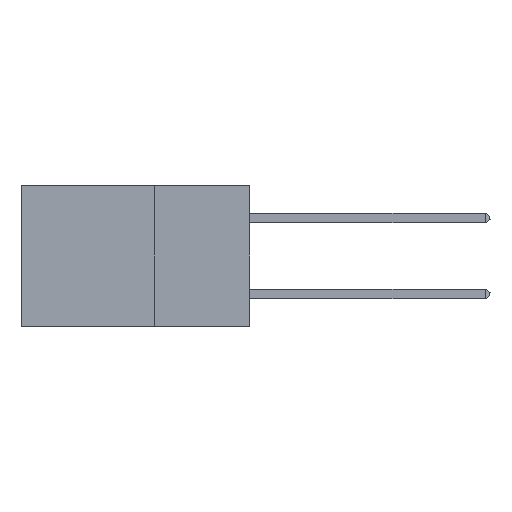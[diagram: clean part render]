
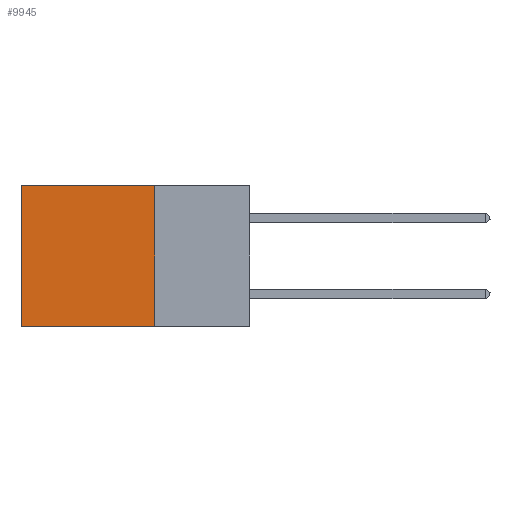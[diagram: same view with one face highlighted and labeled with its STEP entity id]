
A CAD part, left-side view. The second image highlights one B-rep face of the part: STEP entity #9945.
In plain terms, the highlighted planar face has unit normal (-1, 0, 0).
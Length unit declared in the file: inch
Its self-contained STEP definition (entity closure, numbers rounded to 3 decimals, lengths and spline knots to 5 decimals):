
#207 = EDGE_CURVE ( 'NONE', #21221, #17875, #10929, .T. ) ;
#792 = DIRECTION ( 'NONE',  ( 0., 0., -1. ) ) ;
#2050 = AXIS2_PLACEMENT_3D ( 'NONE', #10026, #14637, #792 ) ;
#2463 = ORIENTED_EDGE ( 'NONE', *, *, #19929, .F. ) ;
#3880 = ORIENTED_EDGE ( 'NONE', *, *, #20287, .T. ) ;
#4412 = EDGE_CURVE ( 'NONE', #27515, #17875, #10033, .T. ) ;
#4628 = CARTESIAN_POINT ( 'NONE',  ( 0.2875, 0.6, 0. ) ) ;
#6658 = CARTESIAN_POINT ( 'NONE',  ( 0.2875, 0.25, 0. ) ) ;
#7528 = ORIENTED_EDGE ( 'NONE', *, *, #207, .T. ) ;
#7703 = PLANE ( 'NONE',  #2050 ) ;
#9314 = VECTOR ( 'NONE', #17107, 39.37008 ) ;
#9533 = FACE_OUTER_BOUND ( 'NONE', #23847, .T. ) ;
#9945 = ADVANCED_FACE ( 'NONE', ( #9533 ), #7703, .F. ) ;
#10026 = CARTESIAN_POINT ( 'NONE',  ( 0.2875, 0.25, 0. ) ) ;
#10033 = LINE ( 'NONE', #15262, #15445 ) ;
#10579 = CARTESIAN_POINT ( 'NONE',  ( 0.2875, 0.25, -0.37 ) ) ;
#10929 = LINE ( 'NONE', #4628, #22416 ) ;
#11270 = DIRECTION ( 'NONE',  ( 0., 0., -1. ) ) ;
#12672 = VERTEX_POINT ( 'NONE', #23193 ) ;
#13256 = VECTOR ( 'NONE', #11270, 39.37008 ) ;
#14637 = DIRECTION ( 'NONE',  ( 1., 0., 0. ) ) ;
#15262 = CARTESIAN_POINT ( 'NONE',  ( 0.2875, 0.25, -0.37 ) ) ;
#15445 = VECTOR ( 'NONE', #17542, 39.37008 ) ;
#17107 = DIRECTION ( 'NONE',  ( 0., 1., 0. ) ) ;
#17542 = DIRECTION ( 'NONE',  ( 0., 1., 0. ) ) ;
#17875 = VERTEX_POINT ( 'NONE', #24266 ) ;
#19929 = EDGE_CURVE ( 'NONE', #12672, #27515, #20100, .T. ) ;
#20100 = LINE ( 'NONE', #6658, #13256 ) ;
#20287 = EDGE_CURVE ( 'NONE', #12672, #21221, #21452, .T. ) ;
#20800 = DIRECTION ( 'NONE',  ( 0., 0., -1. ) ) ;
#21221 = VERTEX_POINT ( 'NONE', #26485 ) ;
#21452 = LINE ( 'NONE', #26086, #9314 ) ;
#22416 = VECTOR ( 'NONE', #20800, 39.37008 ) ;
#23193 = CARTESIAN_POINT ( 'NONE',  ( 0.2875, 0.25, 0. ) ) ;
#23847 = EDGE_LOOP ( 'NONE', ( #7528, #23991, #2463, #3880 ) ) ;
#23991 = ORIENTED_EDGE ( 'NONE', *, *, #4412, .F. ) ;
#24266 = CARTESIAN_POINT ( 'NONE',  ( 0.2875, 0.6, -0.37 ) ) ;
#26086 = CARTESIAN_POINT ( 'NONE',  ( 0.2875, 0.25, 0. ) ) ;
#26485 = CARTESIAN_POINT ( 'NONE',  ( 0.2875, 0.6, 0. ) ) ;
#27515 = VERTEX_POINT ( 'NONE', #10579 ) ;
